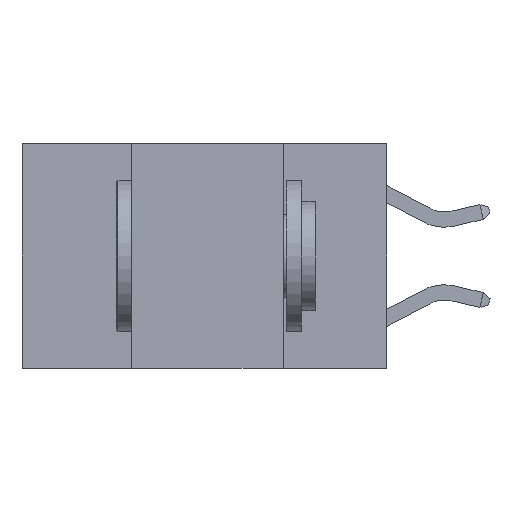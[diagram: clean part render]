
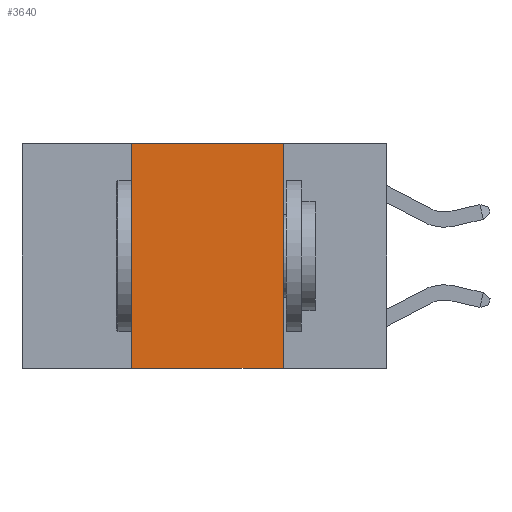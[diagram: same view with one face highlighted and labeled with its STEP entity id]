
A CAD part, left-side view. The second image highlights one B-rep face of the part: STEP entity #3640.
In plain terms, the highlighted planar face has unit normal (-1, 0, 0).
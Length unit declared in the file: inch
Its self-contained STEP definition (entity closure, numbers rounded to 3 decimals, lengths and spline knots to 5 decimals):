
#10 = CARTESIAN_POINT ( 'NONE',  ( 0., 0.17, -0.37 ) ) ;
#1107 = DIRECTION ( 'NONE',  ( 0., -1., 0. ) ) ;
#2472 = CARTESIAN_POINT ( 'NONE',  ( 0., 0.17, 0. ) ) ;
#2621 = EDGE_LOOP ( 'NONE', ( #3414, #16719, #17116, #9297 ) ) ;
#2775 = EDGE_CURVE ( 'NONE', #11444, #17846, #3235, .T. ) ;
#2920 = DIRECTION ( 'NONE',  ( 0., 0., 1. ) ) ;
#2926 = CARTESIAN_POINT ( 'NONE',  ( 0., 0.6, -0.37 ) ) ;
#3062 = EDGE_CURVE ( 'NONE', #12067, #4832, #20312, .T. ) ;
#3235 = LINE ( 'NONE', #7631, #5223 ) ;
#3414 = ORIENTED_EDGE ( 'NONE', *, *, #3062, .F. ) ;
#3640 = ADVANCED_FACE ( 'NONE', ( #17702 ), #12615, .F. ) ;
#4832 = VERTEX_POINT ( 'NONE', #10 ) ;
#5223 = VECTOR ( 'NONE', #2920, 39.37008 ) ;
#6276 = DIRECTION ( 'NONE',  ( 0., -1., 0. ) ) ;
#6359 = LINE ( 'NONE', #2926, #12135 ) ;
#7631 = CARTESIAN_POINT ( 'NONE',  ( 0., 0.42, 0. ) ) ;
#8688 = DIRECTION ( 'NONE',  ( 0., 0., -1. ) ) ;
#8773 = EDGE_CURVE ( 'NONE', #11444, #4832, #6359, .T. ) ;
#9297 = ORIENTED_EDGE ( 'NONE', *, *, #8773, .T. ) ;
#10780 = LINE ( 'NONE', #10988, #14198 ) ;
#10988 = CARTESIAN_POINT ( 'NONE',  ( 0., 0.6, 0. ) ) ;
#11444 = VERTEX_POINT ( 'NONE', #11640 ) ;
#11640 = CARTESIAN_POINT ( 'NONE',  ( 0., 0.42, -0.37 ) ) ;
#12067 = VERTEX_POINT ( 'NONE', #17118 ) ;
#12135 = VECTOR ( 'NONE', #1107, 39.37008 ) ;
#12357 = AXIS2_PLACEMENT_3D ( 'NONE', #12398, #12509, #19108 ) ;
#12398 = CARTESIAN_POINT ( 'NONE',  ( 0., 0.6, 0. ) ) ;
#12509 = DIRECTION ( 'NONE',  ( 1., 0., 0. ) ) ;
#12615 = PLANE ( 'NONE',  #12357 ) ;
#14160 = EDGE_CURVE ( 'NONE', #17846, #12067, #10780, .T. ) ;
#14198 = VECTOR ( 'NONE', #6276, 39.37008 ) ;
#15146 = CARTESIAN_POINT ( 'NONE',  ( 0., 0.42, 0. ) ) ;
#16466 = VECTOR ( 'NONE', #8688, 39.37008 ) ;
#16719 = ORIENTED_EDGE ( 'NONE', *, *, #14160, .F. ) ;
#17116 = ORIENTED_EDGE ( 'NONE', *, *, #2775, .F. ) ;
#17118 = CARTESIAN_POINT ( 'NONE',  ( 0., 0.17, 0. ) ) ;
#17702 = FACE_OUTER_BOUND ( 'NONE', #2621, .T. ) ;
#17846 = VERTEX_POINT ( 'NONE', #15146 ) ;
#19108 = DIRECTION ( 'NONE',  ( 0., 0., -1. ) ) ;
#20312 = LINE ( 'NONE', #2472, #16466 ) ;
